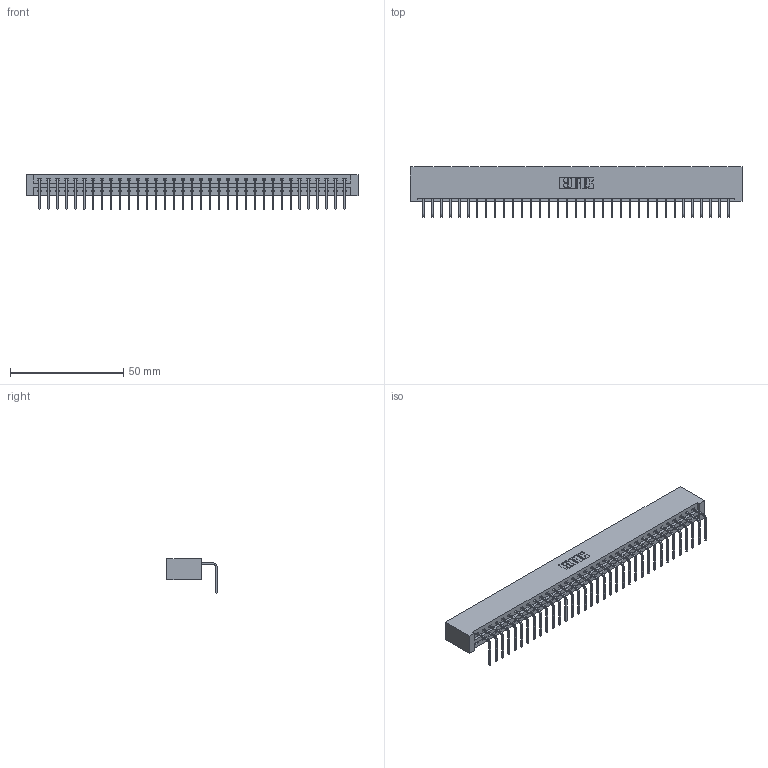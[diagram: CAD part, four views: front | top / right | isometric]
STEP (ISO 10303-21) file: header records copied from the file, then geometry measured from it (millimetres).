
FILE_DESCRIPTION (( 'STEP AP203' ), '1' );
FILE_NAME ('387-035-558-101.STEP', '2018-09-18T22:48:42', ( '' ), ( '' ), 'SwSTEP 2.0', 'SolidWorks 2016', '' );
FILE_SCHEMA (( 'CONFIG_CONTROL_DESIGN' ));
Length unit declared in the file: inch
Products named in the file (3): 337 Part_No Mounting Lugs; 345-292-001_558 Tail - 2; 387-035-558-101
Assembly tree (36 placements, depth 2):
  387-035-558-101
    337 Part_No Mounting Lugs
    345-292-001_558 Tail - 2  x35
Bounding box: 146.56 x 22.17 x 15.37 mm (x, y, z)
Volume: 16000 mm3; surface area: 17192.6 mm2
Topology: 36 solids, 36 shells, 2346 faces, 7077 edges, 4670 vertices
Faces by surface type: plane 1746, cylinder 600
Entity records: 26729 total; most frequent: CARTESIAN_POINT 4663, ORIENTED_EDGE 4634, DIRECTION 3931, EDGE_CURVE 2317, LINE 2197, VECTOR 2197, VERTEX_POINT 1542, AXIS2_PLACEMENT_3D 867
